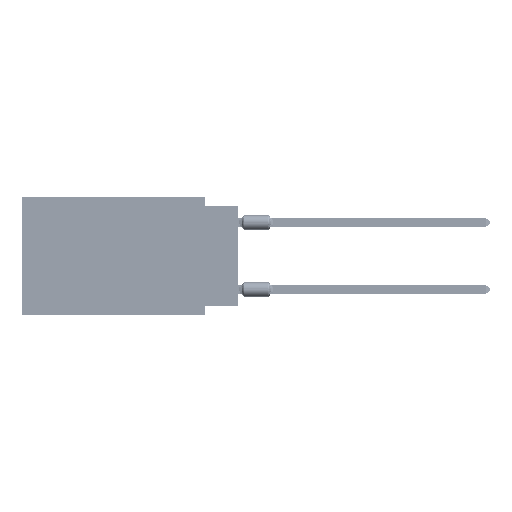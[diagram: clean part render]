
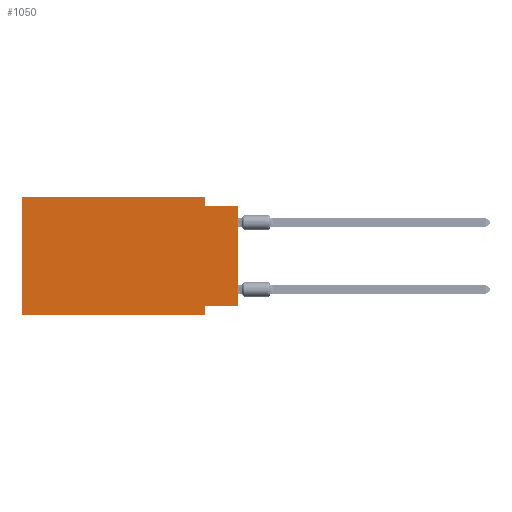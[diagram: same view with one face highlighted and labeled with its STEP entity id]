
A CAD part, left-side view. The second image highlights one B-rep face of the part: STEP entity #1050.
In plain terms, the highlighted planar face has unit normal (-1, 0, 0).
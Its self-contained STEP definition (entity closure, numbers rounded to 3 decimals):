
#1050 = ADVANCED_FACE ( 'NONE', ( #42165 ), #53713, .F. ) ;
#1134 = CARTESIAN_POINT ( 'NONE',  ( 0., 16.383, -8.89 ) ) ;
#1297 = VECTOR ( 'NONE', #38478, 1000. ) ;
#1480 = VECTOR ( 'NONE', #5177, 1000. ) ;
#1732 = VECTOR ( 'NONE', #51064, 1000. ) ;
#3188 = EDGE_CURVE ( 'NONE', #24803, #64534, #32218, .T. ) ;
#4542 = EDGE_CURVE ( 'NONE', #38460, #58686, #8020, .T. ) ;
#5072 = ORIENTED_EDGE ( 'NONE', *, *, #21714, .T. ) ;
#5177 = DIRECTION ( 'NONE',  ( 0., 1., 0. ) ) ;
#5912 = EDGE_CURVE ( 'NONE', #19516, #11019, #51511, .T. ) ;
#6499 = ORIENTED_EDGE ( 'NONE', *, *, #3188, .F. ) ;
#8020 = LINE ( 'NONE', #1134, #1732 ) ;
#8462 = ORIENTED_EDGE ( 'NONE', *, *, #27212, .F. ) ;
#9072 = LINE ( 'NONE', #40560, #25358 ) ;
#9750 = CARTESIAN_POINT ( 'NONE',  ( 0., 0., -0.635 ) ) ;
#11019 = VERTEX_POINT ( 'NONE', #59797 ) ;
#14861 = CARTESIAN_POINT ( 'NONE',  ( 0., 0., 0. ) ) ;
#15027 = DIRECTION ( 'NONE',  ( 0., 0., -1. ) ) ;
#15243 = CARTESIAN_POINT ( 'NONE',  ( 0., 16.383, 0. ) ) ;
#18001 = CARTESIAN_POINT ( 'NONE',  ( 0., 2.54, -8.255 ) ) ;
#18042 = ORIENTED_EDGE ( 'NONE', *, *, #22580, .F. ) ;
#18262 = EDGE_CURVE ( 'NONE', #38460, #19516, #50012, .T. ) ;
#18346 = ORIENTED_EDGE ( 'NONE', *, *, #5912, .F. ) ;
#18993 = VECTOR ( 'NONE', #56295, 1000. ) ;
#19516 = VERTEX_POINT ( 'NONE', #38585 ) ;
#21714 = EDGE_CURVE ( 'NONE', #22114, #64534, #30942, .T. ) ;
#22114 = VERTEX_POINT ( 'NONE', #60166 ) ;
#22580 = EDGE_CURVE ( 'NONE', #22114, #29331, #52413, .T. ) ;
#22738 = CARTESIAN_POINT ( 'NONE',  ( 0., 2.54, -8.89 ) ) ;
#24803 = VERTEX_POINT ( 'NONE', #40283 ) ;
#25358 = VECTOR ( 'NONE', #15027, 1000. ) ;
#27135 = VECTOR ( 'NONE', #62083, 1000. ) ;
#27212 = EDGE_CURVE ( 'NONE', #29331, #58686, #43037, .T. ) ;
#29331 = VERTEX_POINT ( 'NONE', #18001 ) ;
#29363 = CARTESIAN_POINT ( 'NONE',  ( 0., 16.383, 0. ) ) ;
#30617 = ORIENTED_EDGE ( 'NONE', *, *, #4542, .T. ) ;
#30942 = LINE ( 'NONE', #14861, #27135 ) ;
#32218 = LINE ( 'NONE', #38831, #62222 ) ;
#34607 = CARTESIAN_POINT ( 'NONE',  ( 0., 2.54, -8.89 ) ) ;
#34643 = ORIENTED_EDGE ( 'NONE', *, *, #64533, .F. ) ;
#37463 = DIRECTION ( 'NONE',  ( 0., -1., 0. ) ) ;
#38460 = VERTEX_POINT ( 'NONE', #52127 ) ;
#38478 = DIRECTION ( 'NONE',  ( 0., 0., -1. ) ) ;
#38585 = CARTESIAN_POINT ( 'NONE',  ( 0., 16.383, 0. ) ) ;
#38831 = CARTESIAN_POINT ( 'NONE',  ( 0., 0., -0.635 ) ) ;
#40283 = CARTESIAN_POINT ( 'NONE',  ( 0., 2.54, -0.635 ) ) ;
#40313 = DIRECTION ( 'NONE',  ( 0., -1., 0. ) ) ;
#40437 = EDGE_LOOP ( 'NONE', ( #5072, #6499, #34643, #18346, #59974, #30617, #8462, #18042 ) ) ;
#40560 = CARTESIAN_POINT ( 'NONE',  ( 0., 2.54, 0. ) ) ;
#42165 = FACE_OUTER_BOUND ( 'NONE', #40437, .T. ) ;
#43037 = LINE ( 'NONE', #22738, #1297 ) ;
#47858 = CARTESIAN_POINT ( 'NONE',  ( 0., 0., -8.255 ) ) ;
#48116 = DIRECTION ( 'NONE',  ( 0., 0., -1. ) ) ;
#50012 = LINE ( 'NONE', #29363, #18993 ) ;
#51064 = DIRECTION ( 'NONE',  ( 0., -1., 0. ) ) ;
#51082 = VECTOR ( 'NONE', #40313, 1000. ) ;
#51511 = LINE ( 'NONE', #67922, #51082 ) ;
#52127 = CARTESIAN_POINT ( 'NONE',  ( 0., 16.383, -8.89 ) ) ;
#52413 = LINE ( 'NONE', #47858, #1480 ) ;
#53713 = PLANE ( 'NONE',  #61794 ) ;
#56295 = DIRECTION ( 'NONE',  ( 0., 0., 1. ) ) ;
#58686 = VERTEX_POINT ( 'NONE', #34607 ) ;
#59797 = CARTESIAN_POINT ( 'NONE',  ( 0., 2.54, 0. ) ) ;
#59974 = ORIENTED_EDGE ( 'NONE', *, *, #18262, .F. ) ;
#60166 = CARTESIAN_POINT ( 'NONE',  ( 0., 0., -8.255 ) ) ;
#61794 = AXIS2_PLACEMENT_3D ( 'NONE', #15243, #68749, #48116 ) ;
#62083 = DIRECTION ( 'NONE',  ( 0., 0., 1. ) ) ;
#62222 = VECTOR ( 'NONE', #37463, 1000. ) ;
#64533 = EDGE_CURVE ( 'NONE', #11019, #24803, #9072, .T. ) ;
#64534 = VERTEX_POINT ( 'NONE', #9750 ) ;
#67922 = CARTESIAN_POINT ( 'NONE',  ( 0., 16.383, 0. ) ) ;
#68749 = DIRECTION ( 'NONE',  ( 1., 0., 0. ) ) ;
